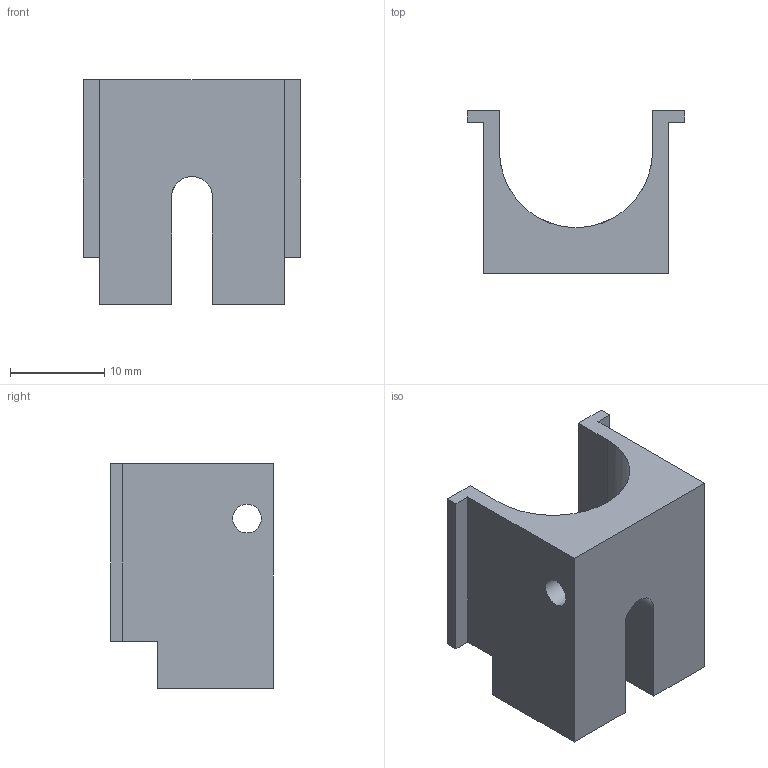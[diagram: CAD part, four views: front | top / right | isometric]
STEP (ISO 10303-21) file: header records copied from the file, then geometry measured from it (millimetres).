
FILE_DESCRIPTION(('FreeCAD Model'),'2;1');
FILE_NAME('GlockRails.step','2020-01-31T16:28:26',( 'Author'),(''),'Open CASCADE STEP processor 6.9','FreeCAD','Unknown' );
FILE_SCHEMA(('AUTOMOTIVE_DESIGN_CC2 { 1 2 10303 214 -1 1 5 4 }'));
Length unit declared in the file: millimetre
Products named in the file (1): Pocket002
Bounding box: 23.11 x 17.27 x 23.88 mm (x, y, z)
Volume: 3492.9 mm3; surface area: 2745.8 mm2
Topology: 1 solids, 1 shells, 23 faces, 65 edges, 44 vertices
Faces by surface type: plane 20, cylinder 3
Full cylindrical faces by diameter (mm): 3.048 x1
Entity records: 1729 total; most frequent: CARTESIAN_POINT 459, DIRECTION 212, LINE 142, VECTOR 142, ORIENTED_EDGE 130, PCURVE 130, DEFINITIONAL_REPRESENTATION 130, EDGE_CURVE 65
